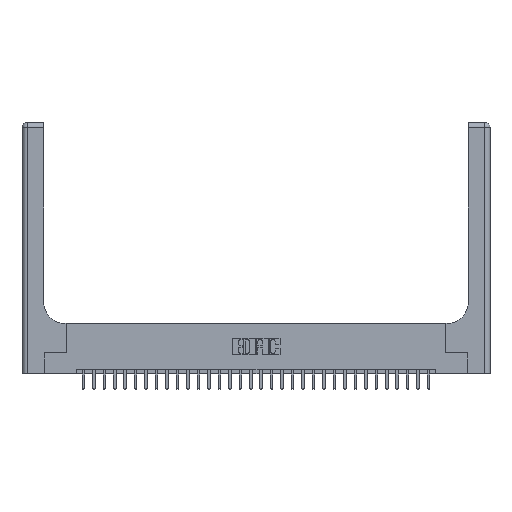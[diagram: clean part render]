
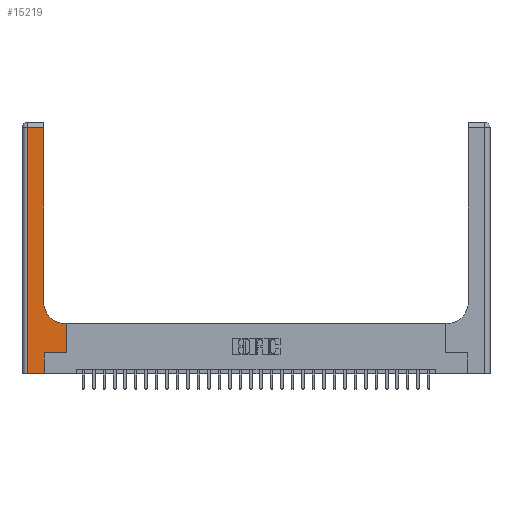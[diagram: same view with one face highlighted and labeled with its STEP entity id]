
A CAD part, top view. The second image highlights one B-rep face of the part: STEP entity #15219.
In plain terms, the highlighted planar face has unit normal (0, 0, 1).
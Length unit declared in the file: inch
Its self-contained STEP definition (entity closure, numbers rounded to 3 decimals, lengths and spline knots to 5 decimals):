
#453 = VERTEX_POINT ( 'NONE', #21025 ) ;
#896 = VERTEX_POINT ( 'NONE', #24555 ) ;
#1461 = CARTESIAN_POINT ( 'NONE',  ( 0.528, 0.25, 0.37 ) ) ;
#1554 = EDGE_CURVE ( 'NONE', #24526, #12490, #14799, .T. ) ;
#1877 = LINE ( 'NONE', #26963, #5015 ) ;
#2679 = ORIENTED_EDGE ( 'NONE', *, *, #22371, .T. ) ;
#2715 = LINE ( 'NONE', #17887, #16506 ) ;
#2858 = CARTESIAN_POINT ( 'NONE',  ( 0.26, 2.94, 0.37 ) ) ;
#3338 = CARTESIAN_POINT ( 'NONE',  ( 0.265, 0.25, 0.37 ) ) ;
#3778 = ORIENTED_EDGE ( 'NONE', *, *, #4369, .T. ) ;
#3828 = AXIS2_PLACEMENT_3D ( 'NONE', #11618, #9331, #21114 ) ;
#4369 = EDGE_CURVE ( 'NONE', #12490, #20411, #5377, .T. ) ;
#4396 = EDGE_CURVE ( 'NONE', #453, #16051, #1877, .T. ) ;
#4559 = DIRECTION ( 'NONE',  ( 0., -1., 0. ) ) ;
#5015 = VECTOR ( 'NONE', #15829, 39.37008 ) ;
#5377 = LINE ( 'NONE', #25717, #17760 ) ;
#5709 = ORIENTED_EDGE ( 'NONE', *, *, #15786, .T. ) ;
#6324 = CARTESIAN_POINT ( 'NONE',  ( 0.265, 0.25, 0.37 ) ) ;
#6602 = CARTESIAN_POINT ( 'NONE',  ( 0.06, 3., 0.37 ) ) ;
#7898 = DIRECTION ( 'NONE',  ( 1., 0., 0. ) ) ;
#9331 = DIRECTION ( 'NONE',  ( 0., 0., -1. ) ) ;
#9332 = CARTESIAN_POINT ( 'NONE',  ( 0.51, 0.85, 0.37 ) ) ;
#9607 = DIRECTION ( 'NONE',  ( -1., 0., 0. ) ) ;
#10139 = EDGE_LOOP ( 'NONE', ( #3778, #20810, #25000, #17882, #18093, #5709, #15032, #2679, #27075 ) ) ;
#10258 = VERTEX_POINT ( 'NONE', #17921 ) ;
#11539 = FACE_OUTER_BOUND ( 'NONE', #10139, .T. ) ;
#11618 = CARTESIAN_POINT ( 'NONE',  ( 0., 3., 0.37 ) ) ;
#12395 = LINE ( 'NONE', #20539, #26229 ) ;
#12490 = VERTEX_POINT ( 'NONE', #28453 ) ;
#13022 = VECTOR ( 'NONE', #15323, 39.37008 ) ;
#14213 = LINE ( 'NONE', #20172, #26673 ) ;
#14799 = CIRCLE ( 'NONE', #16298, 0.25 ) ;
#15032 = ORIENTED_EDGE ( 'NONE', *, *, #20958, .T. ) ;
#15219 = ADVANCED_FACE ( 'NONE', ( #11539 ), #22485, .F. ) ;
#15323 = DIRECTION ( 'NONE',  ( 1., 0., 0. ) ) ;
#15713 = DIRECTION ( 'NONE',  ( 0., 1., 0. ) ) ;
#15786 = EDGE_CURVE ( 'NONE', #16051, #17067, #27373, .T. ) ;
#15829 = DIRECTION ( 'NONE',  ( 0., 1., 0. ) ) ;
#16051 = VERTEX_POINT ( 'NONE', #6324 ) ;
#16298 = AXIS2_PLACEMENT_3D ( 'NONE', #9332, #20463, #18156 ) ;
#16506 = VECTOR ( 'NONE', #24546, 39.37008 ) ;
#16593 = LINE ( 'NONE', #6602, #26261 ) ;
#17067 = VERTEX_POINT ( 'NONE', #1461 ) ;
#17251 = EDGE_CURVE ( 'NONE', #26174, #896, #16593, .T. ) ;
#17627 = CARTESIAN_POINT ( 'NONE',  ( 0.51, 0.6, 0.37 ) ) ;
#17760 = VECTOR ( 'NONE', #22690, 39.37008 ) ;
#17882 = ORIENTED_EDGE ( 'NONE', *, *, #18891, .T. ) ;
#17887 = CARTESIAN_POINT ( 'NONE',  ( 0., 2.94, 0.37 ) ) ;
#17921 = CARTESIAN_POINT ( 'NONE',  ( 0.528, 0.6, 0.37 ) ) ;
#18093 = ORIENTED_EDGE ( 'NONE', *, *, #4396, .T. ) ;
#18156 = DIRECTION ( 'NONE',  ( 1., 0., 0. ) ) ;
#18891 = EDGE_CURVE ( 'NONE', #896, #453, #19557, .T. ) ;
#19557 = LINE ( 'NONE', #24135, #13022 ) ;
#20172 = CARTESIAN_POINT ( 'NONE',  ( 0.528, 0.25, 0.37 ) ) ;
#20411 = VERTEX_POINT ( 'NONE', #2858 ) ;
#20463 = DIRECTION ( 'NONE',  ( 0., 0., -1. ) ) ;
#20539 = CARTESIAN_POINT ( 'NONE',  ( 0.26, 0.6, 0.37 ) ) ;
#20810 = ORIENTED_EDGE ( 'NONE', *, *, #23505, .T. ) ;
#20958 = EDGE_CURVE ( 'NONE', #17067, #10258, #14213, .T. ) ;
#21025 = CARTESIAN_POINT ( 'NONE',  ( 0.265, 0., 0.37 ) ) ;
#21114 = DIRECTION ( 'NONE',  ( -1., 0., 0. ) ) ;
#21229 = CARTESIAN_POINT ( 'NONE',  ( 0.06, 2.94, 0.37 ) ) ;
#22371 = EDGE_CURVE ( 'NONE', #10258, #24526, #12395, .T. ) ;
#22485 = PLANE ( 'NONE',  #3828 ) ;
#22520 = VECTOR ( 'NONE', #7898, 39.37008 ) ;
#22690 = DIRECTION ( 'NONE',  ( 0., 1., 0. ) ) ;
#23505 = EDGE_CURVE ( 'NONE', #20411, #26174, #2715, .T. ) ;
#24135 = CARTESIAN_POINT ( 'NONE',  ( 0., 0., 0.37 ) ) ;
#24526 = VERTEX_POINT ( 'NONE', #17627 ) ;
#24546 = DIRECTION ( 'NONE',  ( -1., 0., 0. ) ) ;
#24555 = CARTESIAN_POINT ( 'NONE',  ( 0.06, 0., 0.37 ) ) ;
#25000 = ORIENTED_EDGE ( 'NONE', *, *, #17251, .T. ) ;
#25717 = CARTESIAN_POINT ( 'NONE',  ( 0.26, 3., 0.37 ) ) ;
#26174 = VERTEX_POINT ( 'NONE', #21229 ) ;
#26229 = VECTOR ( 'NONE', #9607, 39.37008 ) ;
#26261 = VECTOR ( 'NONE', #4559, 39.37008 ) ;
#26673 = VECTOR ( 'NONE', #15713, 39.37008 ) ;
#26963 = CARTESIAN_POINT ( 'NONE',  ( 0.265, 0., 0.37 ) ) ;
#27075 = ORIENTED_EDGE ( 'NONE', *, *, #1554, .T. ) ;
#27373 = LINE ( 'NONE', #3338, #22520 ) ;
#28453 = CARTESIAN_POINT ( 'NONE',  ( 0.26, 0.85, 0.37 ) ) ;
